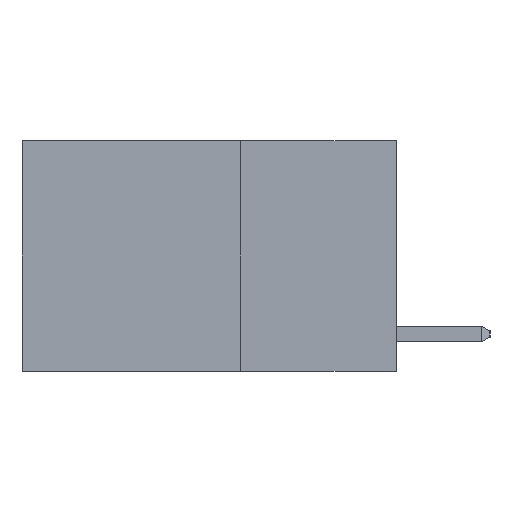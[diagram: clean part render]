
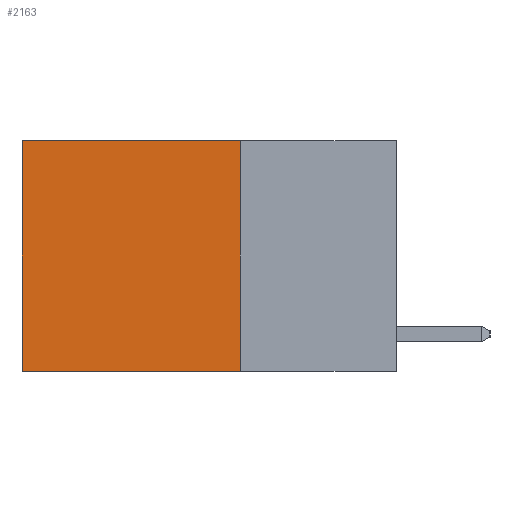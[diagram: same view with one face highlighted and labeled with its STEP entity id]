
A CAD part, left-side view. The second image highlights one B-rep face of the part: STEP entity #2163.
In plain terms, the highlighted planar face has unit normal (-1, 0, 0).
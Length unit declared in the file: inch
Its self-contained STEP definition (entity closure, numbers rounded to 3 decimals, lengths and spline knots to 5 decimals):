
#16 = CARTESIAN_POINT ( 'NONE',  ( 0.2625, 0.25, 0. ) ) ;
#104 = LINE ( 'NONE', #8448, #8991 ) ;
#228 = CARTESIAN_POINT ( 'NONE',  ( 0.2625, 0.25, 0. ) ) ;
#236 = CARTESIAN_POINT ( 'NONE',  ( 0.2625, 0.6, 0. ) ) ;
#689 = ORIENTED_EDGE ( 'NONE', *, *, #1006, .T. ) ;
#994 = FACE_OUTER_BOUND ( 'NONE', #6578, .T. ) ;
#1006 = EDGE_CURVE ( 'NONE', #2366, #4046, #8290, .T. ) ;
#1206 = DIRECTION ( 'NONE',  ( 1., 0., 0. ) ) ;
#1707 = CARTESIAN_POINT ( 'NONE',  ( 0.2625, 0.6, -0.37 ) ) ;
#1911 = ORIENTED_EDGE ( 'NONE', *, *, #5443, .T. ) ;
#2039 = VERTEX_POINT ( 'NONE', #1707 ) ;
#2163 = ADVANCED_FACE ( 'NONE', ( #994 ), #4697, .F. ) ;
#2213 = CARTESIAN_POINT ( 'NONE',  ( 0.2625, 0.6, 0. ) ) ;
#2366 = VERTEX_POINT ( 'NONE', #16 ) ;
#2699 = AXIS2_PLACEMENT_3D ( 'NONE', #5351, #1206, #6030 ) ;
#3285 = CARTESIAN_POINT ( 'NONE',  ( 0.2625, 0.25, -0.37 ) ) ;
#3514 = CARTESIAN_POINT ( 'NONE',  ( 0.2625, 0.25, -0.37 ) ) ;
#3725 = DIRECTION ( 'NONE',  ( 0., 0., -1. ) ) ;
#4046 = VERTEX_POINT ( 'NONE', #2213 ) ;
#4170 = DIRECTION ( 'NONE',  ( 0., 1., 0. ) ) ;
#4211 = DIRECTION ( 'NONE',  ( 0., 1., 0. ) ) ;
#4697 = PLANE ( 'NONE',  #2699 ) ;
#4735 = VECTOR ( 'NONE', #8607, 39.37008 ) ;
#4931 = LINE ( 'NONE', #236, #4735 ) ;
#5351 = CARTESIAN_POINT ( 'NONE',  ( 0.2625, 0.25, 0. ) ) ;
#5370 = ORIENTED_EDGE ( 'NONE', *, *, #7980, .F. ) ;
#5434 = LINE ( 'NONE', #3514, #8881 ) ;
#5443 = EDGE_CURVE ( 'NONE', #4046, #2039, #4931, .T. ) ;
#6030 = DIRECTION ( 'NONE',  ( 0., 0., -1. ) ) ;
#6578 = EDGE_LOOP ( 'NONE', ( #1911, #5370, #7115, #689 ) ) ;
#7115 = ORIENTED_EDGE ( 'NONE', *, *, #7428, .F. ) ;
#7428 = EDGE_CURVE ( 'NONE', #2366, #7738, #104, .T. ) ;
#7738 = VERTEX_POINT ( 'NONE', #3285 ) ;
#7980 = EDGE_CURVE ( 'NONE', #7738, #2039, #5434, .T. ) ;
#8078 = VECTOR ( 'NONE', #4170, 39.37008 ) ;
#8290 = LINE ( 'NONE', #228, #8078 ) ;
#8448 = CARTESIAN_POINT ( 'NONE',  ( 0.2625, 0.25, 0. ) ) ;
#8607 = DIRECTION ( 'NONE',  ( 0., 0., -1. ) ) ;
#8881 = VECTOR ( 'NONE', #4211, 39.37008 ) ;
#8991 = VECTOR ( 'NONE', #3725, 39.37008 ) ;
